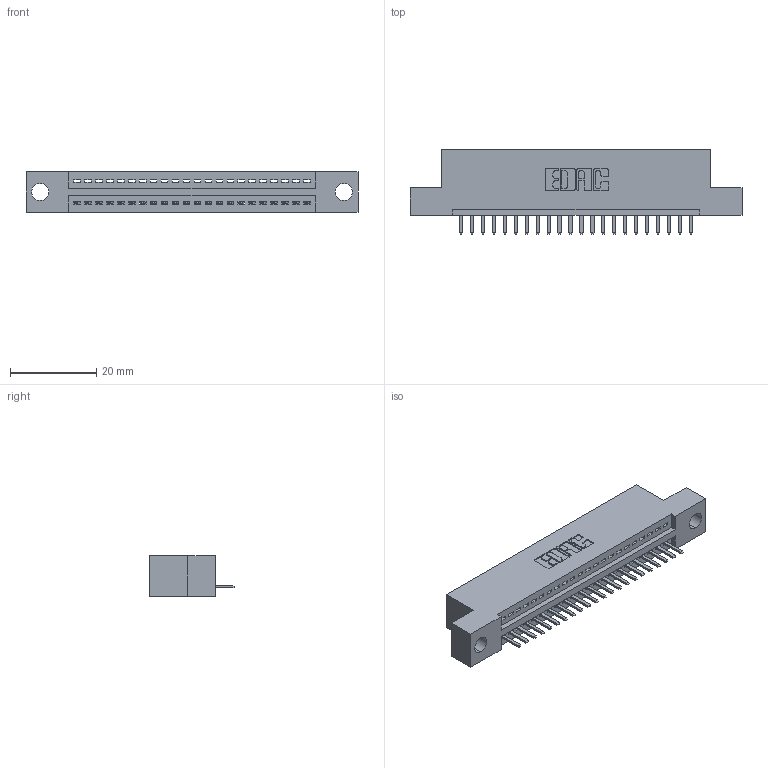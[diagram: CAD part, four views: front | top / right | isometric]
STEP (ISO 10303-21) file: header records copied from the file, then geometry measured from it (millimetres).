
FILE_DESCRIPTION (( 'STEP AP203' ), '1' );
FILE_NAME ('395-022-520-104.STEP', '2018-11-08T00:05:07', ( '' ), ( '' ), 'SwSTEP 2.0', 'SolidWorks 2016', '' );
FILE_SCHEMA (( 'CONFIG_CONTROL_DESIGN' ));
Length unit declared in the file: inch
Products named in the file (3): 345-292-001_345-293-120; 395-022-520-104; 345 Part_Flush Mounting Lugs - 0.156 Dia-TH
Assembly tree (23 placements, depth 2):
  395-022-520-104
    345 Part_Flush Mounting Lugs - 0.156 Dia-TH
    345-292-001_345-293-120  x22
Bounding box: 77.09 x 19.68 x 9.4 mm (x, y, z)
Volume: 7007 mm3; surface area: 8641.6 mm2
Topology: 23 solids, 23 shells, 1490 faces, 4389 edges, 2866 vertices
Faces by surface type: plane 1004, cylinder 486
Entity records: 19367 total; most frequent: CARTESIAN_POINT 3374, ORIENTED_EDGE 3318, DIRECTION 2963, EDGE_CURVE 1659, LINE 1435, VECTOR 1435, VERTEX_POINT 1102, AXIS2_PLACEMENT_3D 764
